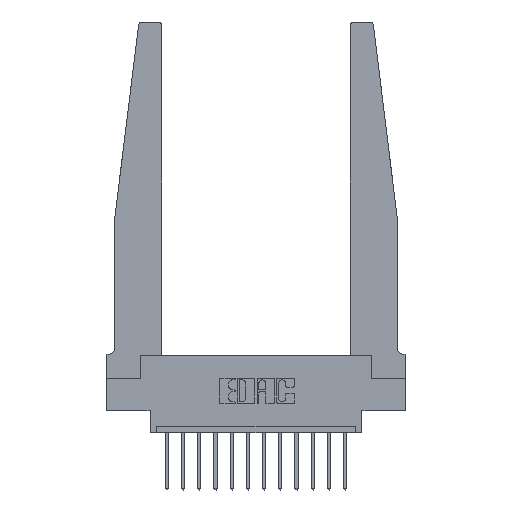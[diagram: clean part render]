
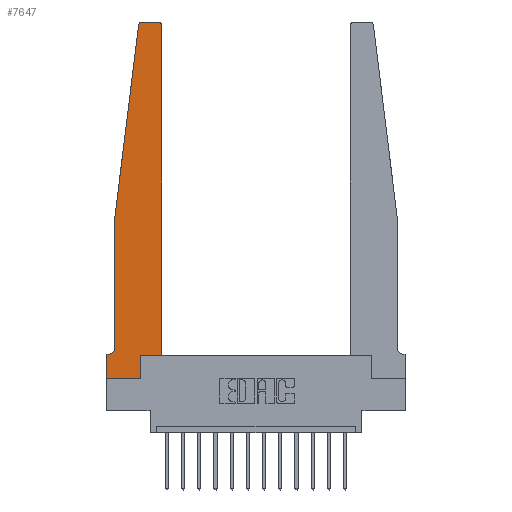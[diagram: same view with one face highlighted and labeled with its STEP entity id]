
A CAD part, top view. The second image highlights one B-rep face of the part: STEP entity #7647.
In plain terms, the highlighted planar face has unit normal (0, 0, 1).
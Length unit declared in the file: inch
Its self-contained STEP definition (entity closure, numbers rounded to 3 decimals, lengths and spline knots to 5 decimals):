
#272 = CARTESIAN_POINT ( 'NONE',  ( 0.425, 0.18, 0.37 ) ) ;
#988 = CARTESIAN_POINT ( 'NONE',  ( 0., 0., 0.37 ) ) ;
#1030 = CARTESIAN_POINT ( 'NONE',  ( 0.2605, 0.18, 0.37 ) ) ;
#1153 = ORIENTED_EDGE ( 'NONE', *, *, #1456, .T. ) ;
#1323 = LINE ( 'NONE', #6511, #15988 ) ;
#1456 = EDGE_CURVE ( 'NONE', #15603, #11821, #8491, .T. ) ;
#1541 = LINE ( 'NONE', #272, #1882 ) ;
#1559 = AXIS2_PLACEMENT_3D ( 'NONE', #1560, #14593, #4200 ) ;
#1560 = CARTESIAN_POINT ( 'NONE',  ( 0.015, 0.2375, 0.37 ) ) ;
#1616 = VECTOR ( 'NONE', #16709, 39.37008 ) ;
#1630 = VECTOR ( 'NONE', #6630, 39.37008 ) ;
#1845 = LINE ( 'NONE', #13524, #2602 ) ;
#1882 = VECTOR ( 'NONE', #10682, 39.37008 ) ;
#1893 = CARTESIAN_POINT ( 'NONE',  ( 0.27653, 2.75, 0.37 ) ) ;
#2105 = ORIENTED_EDGE ( 'NONE', *, *, #14983, .T. ) ;
#2123 = EDGE_CURVE ( 'NONE', #15954, #5322, #5537, .T. ) ;
#2287 = DIRECTION ( 'NONE',  ( 1., 0., 0. ) ) ;
#2310 = VERTEX_POINT ( 'NONE', #11687 ) ;
#2602 = VECTOR ( 'NONE', #3125, 39.37008 ) ;
#2924 = CARTESIAN_POINT ( 'NONE',  ( 0.065, 0.1875, 0.37 ) ) ;
#3061 = VECTOR ( 'NONE', #13134, 39.37008 ) ;
#3125 = DIRECTION ( 'NONE',  ( -1., 0., 0. ) ) ;
#3430 = CARTESIAN_POINT ( 'NONE',  ( 0.065, 1.25, 0.37 ) ) ;
#4084 = CARTESIAN_POINT ( 'NONE',  ( 0.065, 1.25, 0.37 ) ) ;
#4200 = DIRECTION ( 'NONE',  ( -1., 0., 0. ) ) ;
#4205 = DIRECTION ( 'NONE',  ( -1., 0., 0. ) ) ;
#4465 = EDGE_CURVE ( 'NONE', #2310, #13558, #16758, .T. ) ;
#4492 = CARTESIAN_POINT ( 'NONE',  ( 0.395, 2.75, 0.37 ) ) ;
#4513 = CARTESIAN_POINT ( 'NONE',  ( 0., 0., 0.37 ) ) ;
#4750 = CARTESIAN_POINT ( 'NONE',  ( 0.27653, 2.72, 0.37 ) ) ;
#4983 = ORIENTED_EDGE ( 'NONE', *, *, #8009, .T. ) ;
#5322 = VERTEX_POINT ( 'NONE', #4513 ) ;
#5537 = LINE ( 'NONE', #7951, #3061 ) ;
#6511 = CARTESIAN_POINT ( 'NONE',  ( 0.2605, 0.18, 0.37 ) ) ;
#6606 = EDGE_CURVE ( 'NONE', #12503, #15603, #1323, .T. ) ;
#6630 = DIRECTION ( 'NONE',  ( 0., -1., 0. ) ) ;
#6886 = EDGE_CURVE ( 'NONE', #16045, #2310, #7257, .T. ) ;
#7001 = CARTESIAN_POINT ( 'NONE',  ( 0., 0.1875, 0.37 ) ) ;
#7018 = CARTESIAN_POINT ( 'NONE',  ( 0.015, 0.1875, 0.37 ) ) ;
#7257 = LINE ( 'NONE', #3430, #15484 ) ;
#7366 = LINE ( 'NONE', #988, #16497 ) ;
#7425 = ORIENTED_EDGE ( 'NONE', *, *, #4465, .T. ) ;
#7647 = ADVANCED_FACE ( 'NONE', ( #13570 ), #9570, .T. ) ;
#7735 = VERTEX_POINT ( 'NONE', #1893 ) ;
#7951 = CARTESIAN_POINT ( 'NONE',  ( 0., 0., 0.37 ) ) ;
#8009 = EDGE_CURVE ( 'NONE', #9356, #7735, #1845, .T. ) ;
#8128 = EDGE_CURVE ( 'NONE', #14668, #9356, #13491, .T. ) ;
#8249 = ORIENTED_EDGE ( 'NONE', *, *, #6886, .T. ) ;
#8422 = DIRECTION ( 'NONE',  ( 0., 0., 1. ) ) ;
#8491 = LINE ( 'NONE', #13678, #1616 ) ;
#8495 = VERTEX_POINT ( 'NONE', #7018 ) ;
#8758 = DIRECTION ( 'NONE',  ( 0., 0., 1. ) ) ;
#9198 = AXIS2_PLACEMENT_3D ( 'NONE', #7001, #12386, #16190 ) ;
#9356 = VERTEX_POINT ( 'NONE', #4492 ) ;
#9570 = PLANE ( 'NONE',  #9198 ) ;
#9600 = CARTESIAN_POINT ( 'NONE',  ( 0.24675, 2.72367, 0.37 ) ) ;
#9809 = EDGE_CURVE ( 'NONE', #5322, #12503, #7366, .T. ) ;
#10682 = DIRECTION ( 'NONE',  ( 0., 1., 0. ) ) ;
#10835 = CIRCLE ( 'NONE', #1559, 0.05 ) ;
#10973 = CARTESIAN_POINT ( 'NONE',  ( 0.425, 0.18, 0.37 ) ) ;
#11330 = AXIS2_PLACEMENT_3D ( 'NONE', #16068, #8422, #12345 ) ;
#11676 = CARTESIAN_POINT ( 'NONE',  ( 0., 0.1875, 0.37 ) ) ;
#11683 = CIRCLE ( 'NONE', #16273, 0.03 ) ;
#11687 = CARTESIAN_POINT ( 'NONE',  ( 0.065, 1.25, 0.37 ) ) ;
#11774 = ORIENTED_EDGE ( 'NONE', *, *, #13804, .T. ) ;
#11821 = VERTEX_POINT ( 'NONE', #10973 ) ;
#12084 = CARTESIAN_POINT ( 'NONE',  ( 0.425, 2.72, 0.37 ) ) ;
#12130 = EDGE_CURVE ( 'NONE', #13558, #8495, #10835, .T. ) ;
#12345 = DIRECTION ( 'NONE',  ( 1., 0., 0. ) ) ;
#12386 = DIRECTION ( 'NONE',  ( 0., 0., 1. ) ) ;
#12503 = VERTEX_POINT ( 'NONE', #13552 ) ;
#12742 = DIRECTION ( 'NONE',  ( 0., 1., 0. ) ) ;
#12756 = ORIENTED_EDGE ( 'NONE', *, *, #12130, .T. ) ;
#13127 = EDGE_CURVE ( 'NONE', #7735, #16045, #11683, .T. ) ;
#13134 = DIRECTION ( 'NONE',  ( 0., -1., 0. ) ) ;
#13245 = LINE ( 'NONE', #2924, #15232 ) ;
#13358 = ORIENTED_EDGE ( 'NONE', *, *, #9809, .T. ) ;
#13491 = CIRCLE ( 'NONE', #11330, 0.03 ) ;
#13524 = CARTESIAN_POINT ( 'NONE',  ( 0.25, 2.75, 0.37 ) ) ;
#13552 = CARTESIAN_POINT ( 'NONE',  ( 0.2605, 0., 0.37 ) ) ;
#13558 = VERTEX_POINT ( 'NONE', #16781 ) ;
#13570 = FACE_OUTER_BOUND ( 'NONE', #14262, .T. ) ;
#13678 = CARTESIAN_POINT ( 'NONE',  ( 0.425, 0.18, 0.37 ) ) ;
#13804 = EDGE_CURVE ( 'NONE', #11821, #14668, #1541, .T. ) ;
#14262 = EDGE_LOOP ( 'NONE', ( #4983, #14832, #8249, #7425, #12756, #2105, #15536, #13358, #16013, #1153, #11774, #15355 ) ) ;
#14593 = DIRECTION ( 'NONE',  ( 0., 0., -1. ) ) ;
#14668 = VERTEX_POINT ( 'NONE', #12084 ) ;
#14832 = ORIENTED_EDGE ( 'NONE', *, *, #13127, .T. ) ;
#14983 = EDGE_CURVE ( 'NONE', #8495, #15954, #13245, .T. ) ;
#15232 = VECTOR ( 'NONE', #4205, 39.37008 ) ;
#15278 = DIRECTION ( 'NONE',  ( 1., 0., 0. ) ) ;
#15355 = ORIENTED_EDGE ( 'NONE', *, *, #8128, .T. ) ;
#15484 = VECTOR ( 'NONE', #16195, 39.37008 ) ;
#15536 = ORIENTED_EDGE ( 'NONE', *, *, #2123, .T. ) ;
#15603 = VERTEX_POINT ( 'NONE', #1030 ) ;
#15954 = VERTEX_POINT ( 'NONE', #11676 ) ;
#15988 = VECTOR ( 'NONE', #12742, 39.37008 ) ;
#16013 = ORIENTED_EDGE ( 'NONE', *, *, #6606, .T. ) ;
#16045 = VERTEX_POINT ( 'NONE', #9600 ) ;
#16068 = CARTESIAN_POINT ( 'NONE',  ( 0.395, 2.72, 0.37 ) ) ;
#16190 = DIRECTION ( 'NONE',  ( 1., 0., 0. ) ) ;
#16195 = DIRECTION ( 'NONE',  ( -0.122, -0.992, 0. ) ) ;
#16273 = AXIS2_PLACEMENT_3D ( 'NONE', #4750, #8758, #2287 ) ;
#16497 = VECTOR ( 'NONE', #15278, 39.37008 ) ;
#16709 = DIRECTION ( 'NONE',  ( 1., 0., 0. ) ) ;
#16758 = LINE ( 'NONE', #4084, #1630 ) ;
#16781 = CARTESIAN_POINT ( 'NONE',  ( 0.065, 0.2375, 0.37 ) ) ;
